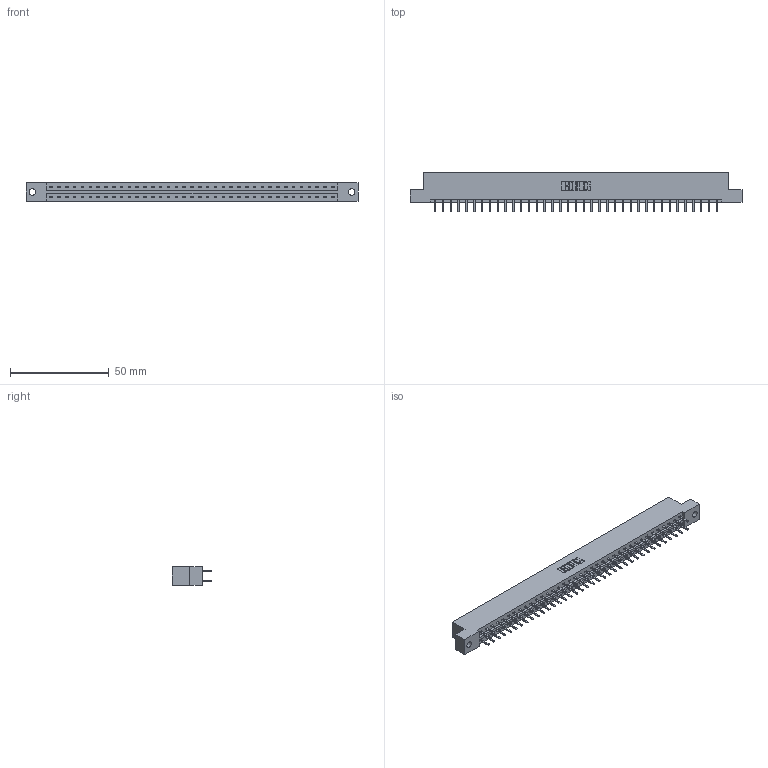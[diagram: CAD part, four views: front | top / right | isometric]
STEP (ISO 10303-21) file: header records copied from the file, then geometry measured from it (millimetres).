
FILE_DESCRIPTION (( 'STEP AP203' ), '1' );
FILE_NAME ('833-074-520-202.STEP', '2020-06-05T15:30:30', ( '' ), ( '' ), 'SwSTEP 2.0', 'SolidWorks 2020', '' );
FILE_SCHEMA (( 'CONFIG_CONTROL_DESIGN' ));
Length unit declared in the file: inch
Products named in the file (3): 345-292-001_345-293-120; 833 Part_Flush - .128 Dia; 833-074-520-202
Assembly tree (75 placements, depth 2):
  833-074-520-202
    833 Part_Flush - .128 Dia
    345-292-001_345-293-120  x74
Bounding box: 168.15 x 20.02 x 9.4 mm (x, y, z)
Volume: 17051 mm3; surface area: 19745.3 mm2
Topology: 75 solids, 75 shells, 4258 faces, 12373 edges, 8050 vertices
Faces by surface type: plane 2882, cylinder 1376
Entity records: 24567 total; most frequent: CARTESIAN_POINT 4090, ORIENTED_EDGE 4014, DIRECTION 3491, EDGE_CURVE 2007, LINE 1875, VECTOR 1875, VERTEX_POINT 1334, AXIS2_PLACEMENT_3D 808
